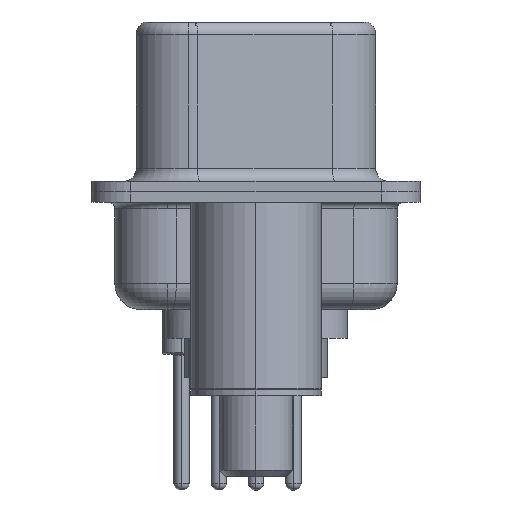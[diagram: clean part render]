
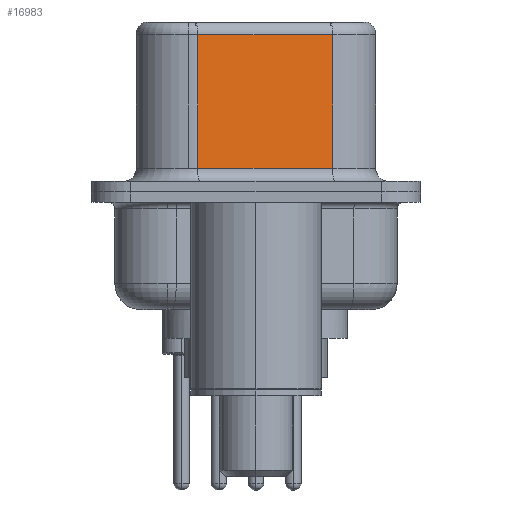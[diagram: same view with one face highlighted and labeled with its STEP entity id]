
A CAD part, left-side view. The second image highlights one B-rep face of the part: STEP entity #16983.
In plain terms, the highlighted planar face has unit normal (-0.985, -0.174, 0).
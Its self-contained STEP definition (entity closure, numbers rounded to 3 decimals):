
#67 = CARTESIAN_POINT ( 'NONE',  ( 3.67, 2.233, 6.02 ) ) ;
#124 = DIRECTION ( 'NONE',  ( -0.174, 0.985, 0. ) ) ;
#167 = CARTESIAN_POINT ( 'NONE',  ( 3.67, 2.233, 0.9 ) ) ;
#357 = VECTOR ( 'NONE', #9291, 1000. ) ;
#2085 = VERTEX_POINT ( 'NONE', #5074 ) ;
#2091 = VECTOR ( 'NONE', #19356, 1000. ) ;
#4040 = EDGE_LOOP ( 'NONE', ( #16093, #4802, #16530, #15325 ) ) ;
#4802 = ORIENTED_EDGE ( 'NONE', *, *, #8115, .T. ) ;
#5074 = CARTESIAN_POINT ( 'NONE',  ( 4.58, -2.927, 0.9 ) ) ;
#6028 = VECTOR ( 'NONE', #15837, 1000. ) ;
#6308 = LINE ( 'NONE', #9586, #2091 ) ;
#7642 = CARTESIAN_POINT ( 'NONE',  ( 4.58, -2.927, 6.52 ) ) ;
#8081 = PLANE ( 'NONE',  #10849 ) ;
#8115 = EDGE_CURVE ( 'NONE', #16271, #11109, #8858, .T. ) ;
#8858 = LINE ( 'NONE', #9734, #357 ) ;
#8914 = EDGE_CURVE ( 'NONE', #16271, #2085, #20601, .T. ) ;
#9291 = DIRECTION ( 'NONE',  ( -0.174, 0.985, 0. ) ) ;
#9586 = CARTESIAN_POINT ( 'NONE',  ( 4.58, -2.927, 0.9 ) ) ;
#9719 = DIRECTION ( 'NONE',  ( 0.985, 0.174, 0. ) ) ;
#9734 = CARTESIAN_POINT ( 'NONE',  ( 4.58, -2.927, 6.02 ) ) ;
#9910 = EDGE_CURVE ( 'NONE', #11109, #20398, #20909, .T. ) ;
#10849 = AXIS2_PLACEMENT_3D ( 'NONE', #17843, #9719, #124 ) ;
#11083 = EDGE_CURVE ( 'NONE', #20398, #2085, #6308, .T. ) ;
#11109 = VERTEX_POINT ( 'NONE', #67 ) ;
#14560 = DIRECTION ( 'NONE',  ( 0., 0., -1. ) ) ;
#14866 = FACE_OUTER_BOUND ( 'NONE', #4040, .T. ) ;
#15325 = ORIENTED_EDGE ( 'NONE', *, *, #11083, .T. ) ;
#15837 = DIRECTION ( 'NONE',  ( 0., 0., -1. ) ) ;
#16093 = ORIENTED_EDGE ( 'NONE', *, *, #8914, .F. ) ;
#16136 = CARTESIAN_POINT ( 'NONE',  ( 3.67, 2.233, 6.52 ) ) ;
#16271 = VERTEX_POINT ( 'NONE', #20978 ) ;
#16530 = ORIENTED_EDGE ( 'NONE', *, *, #9910, .T. ) ;
#16983 = ADVANCED_FACE ( 'NONE', ( #14866 ), #8081, .F. ) ;
#17843 = CARTESIAN_POINT ( 'NONE',  ( 4.58, -2.927, 6.52 ) ) ;
#19356 = DIRECTION ( 'NONE',  ( 0.174, -0.985, 0. ) ) ;
#20398 = VERTEX_POINT ( 'NONE', #167 ) ;
#20401 = VECTOR ( 'NONE', #14560, 1000. ) ;
#20601 = LINE ( 'NONE', #7642, #6028 ) ;
#20909 = LINE ( 'NONE', #16136, #20401 ) ;
#20978 = CARTESIAN_POINT ( 'NONE',  ( 4.58, -2.927, 6.02 ) ) ;
